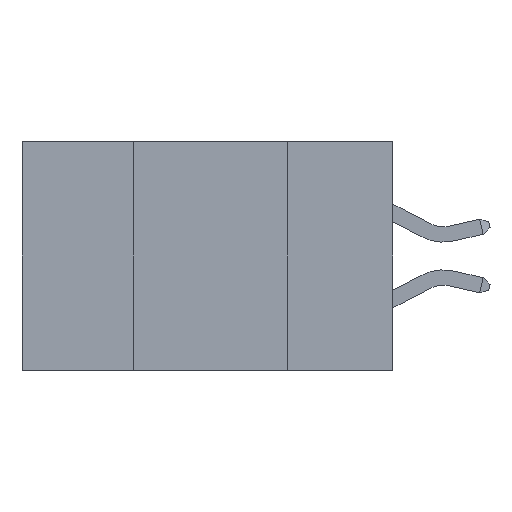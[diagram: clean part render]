
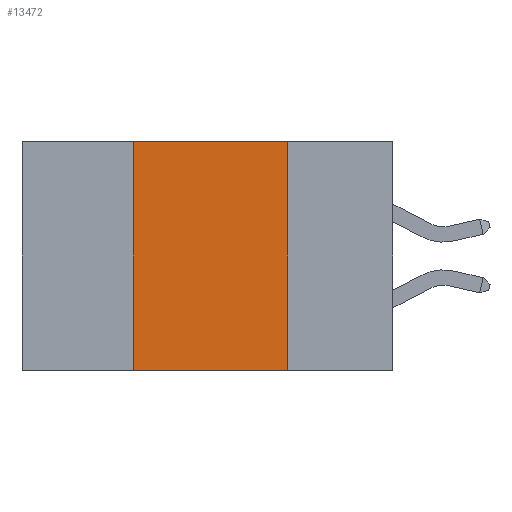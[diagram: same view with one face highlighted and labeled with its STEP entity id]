
A CAD part, left-side view. The second image highlights one B-rep face of the part: STEP entity #13472.
In plain terms, the highlighted planar face has unit normal (-1, 0, 0).
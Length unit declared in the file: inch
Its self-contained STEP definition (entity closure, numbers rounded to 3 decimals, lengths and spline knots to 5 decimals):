
#393 = DIRECTION ( 'NONE',  ( 0., -1., 0. ) ) ;
#588 = VERTEX_POINT ( 'NONE', #21903 ) ;
#1144 = LINE ( 'NONE', #19852, #15589 ) ;
#1244 = ORIENTED_EDGE ( 'NONE', *, *, #21784, .F. ) ;
#2158 = LINE ( 'NONE', #8296, #19275 ) ;
#2487 = CARTESIAN_POINT ( 'NONE',  ( 0., 0.6, 0. ) ) ;
#3922 = CARTESIAN_POINT ( 'NONE',  ( 0., 0.17, 0. ) ) ;
#6480 = CARTESIAN_POINT ( 'NONE',  ( 0., 0.17, 0. ) ) ;
#6850 = FACE_OUTER_BOUND ( 'NONE', #16858, .T. ) ;
#7185 = ORIENTED_EDGE ( 'NONE', *, *, #19829, .T. ) ;
#7344 = DIRECTION ( 'NONE',  ( 0., 0., -1. ) ) ;
#8296 = CARTESIAN_POINT ( 'NONE',  ( 0., 0.6, 0. ) ) ;
#9407 = DIRECTION ( 'NONE',  ( 1., 0., 0. ) ) ;
#9789 = VERTEX_POINT ( 'NONE', #6480 ) ;
#11555 = DIRECTION ( 'NONE',  ( 0., 0., 1. ) ) ;
#12466 = ORIENTED_EDGE ( 'NONE', *, *, #17290, .F. ) ;
#13080 = CARTESIAN_POINT ( 'NONE',  ( 0., 0.17, -0.37 ) ) ;
#13472 = ADVANCED_FACE ( 'NONE', ( #6850 ), #15946, .F. ) ;
#13751 = VERTEX_POINT ( 'NONE', #16553 ) ;
#14266 = CARTESIAN_POINT ( 'NONE',  ( 0., 0.6, -0.37 ) ) ;
#15159 = LINE ( 'NONE', #14266, #16507 ) ;
#15181 = EDGE_CURVE ( 'NONE', #9789, #21678, #19938, .T. ) ;
#15552 = DIRECTION ( 'NONE',  ( 0., -1., 0. ) ) ;
#15589 = VECTOR ( 'NONE', #11555, 39.37008 ) ;
#15946 = PLANE ( 'NONE',  #19863 ) ;
#16507 = VECTOR ( 'NONE', #393, 39.37008 ) ;
#16553 = CARTESIAN_POINT ( 'NONE',  ( 0., 0.42, 0. ) ) ;
#16858 = EDGE_LOOP ( 'NONE', ( #18513, #12466, #1244, #7185 ) ) ;
#17290 = EDGE_CURVE ( 'NONE', #13751, #9789, #2158, .T. ) ;
#18069 = VECTOR ( 'NONE', #7344, 39.37008 ) ;
#18513 = ORIENTED_EDGE ( 'NONE', *, *, #15181, .F. ) ;
#19275 = VECTOR ( 'NONE', #15552, 39.37008 ) ;
#19820 = DIRECTION ( 'NONE',  ( 0., 0., -1. ) ) ;
#19829 = EDGE_CURVE ( 'NONE', #588, #21678, #15159, .T. ) ;
#19852 = CARTESIAN_POINT ( 'NONE',  ( 0., 0.42, 0. ) ) ;
#19863 = AXIS2_PLACEMENT_3D ( 'NONE', #2487, #9407, #19820 ) ;
#19938 = LINE ( 'NONE', #3922, #18069 ) ;
#21678 = VERTEX_POINT ( 'NONE', #13080 ) ;
#21784 = EDGE_CURVE ( 'NONE', #588, #13751, #1144, .T. ) ;
#21903 = CARTESIAN_POINT ( 'NONE',  ( 0., 0.42, -0.37 ) ) ;
